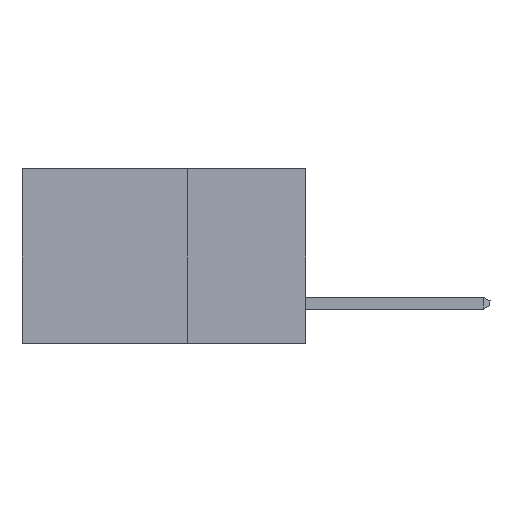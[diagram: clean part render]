
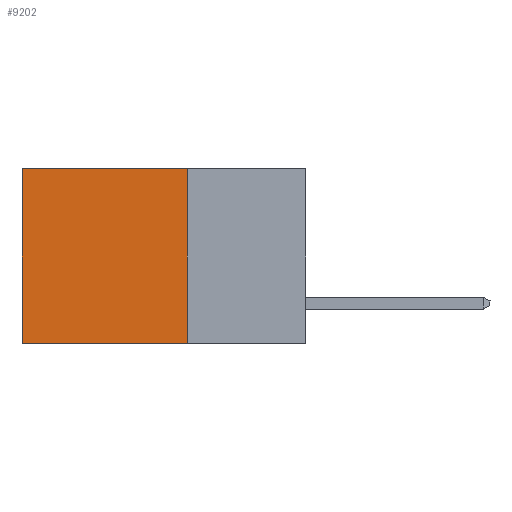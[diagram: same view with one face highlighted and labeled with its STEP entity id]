
A CAD part, left-side view. The second image highlights one B-rep face of the part: STEP entity #9202.
In plain terms, the highlighted planar face has unit normal (-1, 0, 0).
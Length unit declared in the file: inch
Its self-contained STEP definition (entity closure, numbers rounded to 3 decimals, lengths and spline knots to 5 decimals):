
#91 = DIRECTION ( 'NONE',  ( 1., 0., 0. ) ) ;
#187 = VERTEX_POINT ( 'NONE', #4223 ) ;
#286 = VECTOR ( 'NONE', #8788, 39.37008 ) ;
#662 = AXIS2_PLACEMENT_3D ( 'NONE', #7801, #91, #5511 ) ;
#1297 = CARTESIAN_POINT ( 'NONE',  ( 0.2615, 0.25, -0.37 ) ) ;
#1466 = VECTOR ( 'NONE', #8179, 39.37008 ) ;
#1539 = EDGE_LOOP ( 'NONE', ( #7583, #6822, #5212, #3693 ) ) ;
#1653 = CARTESIAN_POINT ( 'NONE',  ( 0.2615, 0.25, -0.37 ) ) ;
#1976 = LINE ( 'NONE', #5074, #1466 ) ;
#2419 = FACE_OUTER_BOUND ( 'NONE', #1539, .T. ) ;
#3293 = CARTESIAN_POINT ( 'NONE',  ( 0.2615, 0.25, 0. ) ) ;
#3693 = ORIENTED_EDGE ( 'NONE', *, *, #5665, .T. ) ;
#3710 = VERTEX_POINT ( 'NONE', #1297 ) ;
#3799 = LINE ( 'NONE', #6893, #4171 ) ;
#3939 = PLANE ( 'NONE',  #662 ) ;
#4171 = VECTOR ( 'NONE', #9997, 39.37008 ) ;
#4223 = CARTESIAN_POINT ( 'NONE',  ( 0.2615, 0.25, 0. ) ) ;
#4743 = DIRECTION ( 'NONE',  ( 0., 1., 0. ) ) ;
#5074 = CARTESIAN_POINT ( 'NONE',  ( 0.2615, 0.6, -0.37 ) ) ;
#5123 = CARTESIAN_POINT ( 'NONE',  ( 0.2615, 0.6, 0. ) ) ;
#5212 = ORIENTED_EDGE ( 'NONE', *, *, #6060, .F. ) ;
#5380 = VERTEX_POINT ( 'NONE', #5123 ) ;
#5511 = DIRECTION ( 'NONE',  ( 0., 0., -1. ) ) ;
#5665 = EDGE_CURVE ( 'NONE', #187, #5380, #7051, .T. ) ;
#6060 = EDGE_CURVE ( 'NONE', #187, #3710, #3799, .T. ) ;
#6324 = VECTOR ( 'NONE', #4743, 39.37008 ) ;
#6822 = ORIENTED_EDGE ( 'NONE', *, *, #9206, .F. ) ;
#6893 = CARTESIAN_POINT ( 'NONE',  ( 0.2615, 0.25, -0.37 ) ) ;
#7051 = LINE ( 'NONE', #3293, #286 ) ;
#7583 = ORIENTED_EDGE ( 'NONE', *, *, #8534, .T. ) ;
#7801 = CARTESIAN_POINT ( 'NONE',  ( 0.2615, 0.25, -0.37 ) ) ;
#8179 = DIRECTION ( 'NONE',  ( 0., 0., -1. ) ) ;
#8190 = VERTEX_POINT ( 'NONE', #8867 ) ;
#8534 = EDGE_CURVE ( 'NONE', #5380, #8190, #1976, .T. ) ;
#8626 = LINE ( 'NONE', #1653, #6324 ) ;
#8788 = DIRECTION ( 'NONE',  ( 0., 1., 0. ) ) ;
#8867 = CARTESIAN_POINT ( 'NONE',  ( 0.2615, 0.6, -0.37 ) ) ;
#9202 = ADVANCED_FACE ( 'NONE', ( #2419 ), #3939, .F. ) ;
#9206 = EDGE_CURVE ( 'NONE', #3710, #8190, #8626, .T. ) ;
#9997 = DIRECTION ( 'NONE',  ( 0., 0., -1. ) ) ;
